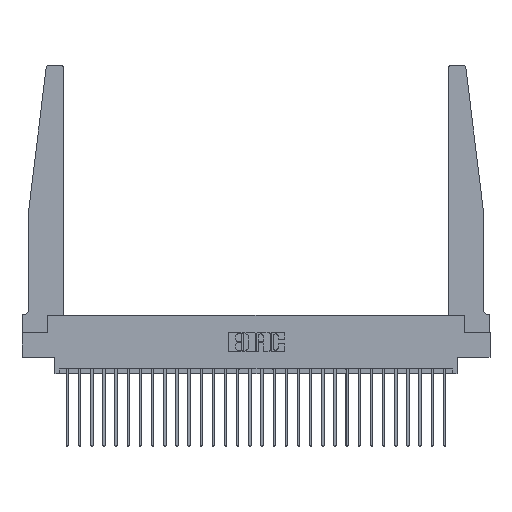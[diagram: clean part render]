
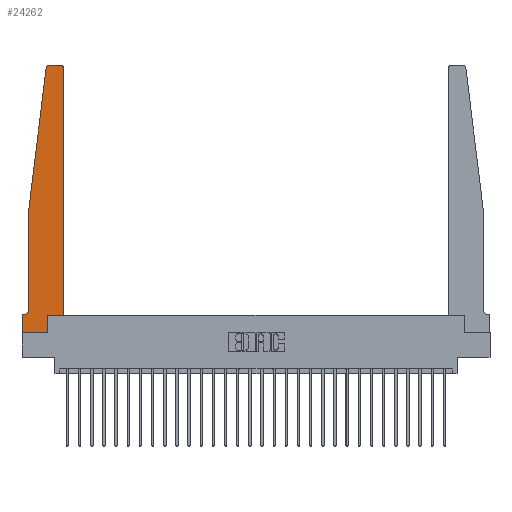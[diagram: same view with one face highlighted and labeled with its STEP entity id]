
A CAD part, top view. The second image highlights one B-rep face of the part: STEP entity #24262.
In plain terms, the highlighted planar face has unit normal (0, 0, 1).
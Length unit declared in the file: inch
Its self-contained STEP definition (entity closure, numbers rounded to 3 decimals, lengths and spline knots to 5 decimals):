
#16 = VECTOR ( 'NONE', #968, 39.37008 ) ;
#245 = ORIENTED_EDGE ( 'NONE', *, *, #18669, .T. ) ;
#570 = CARTESIAN_POINT ( 'NONE',  ( 0., 0.1875, 0.37 ) ) ;
#968 = DIRECTION ( 'NONE',  ( -1., 0., 0. ) ) ;
#1078 = DIRECTION ( 'NONE',  ( 0., 0., 1. ) ) ;
#1541 = EDGE_CURVE ( 'NONE', #19103, #9141, #2400, .T. ) ;
#1894 = AXIS2_PLACEMENT_3D ( 'NONE', #19798, #25999, #13683 ) ;
#2400 = CIRCLE ( 'NONE', #21266, 0.03 ) ;
#2413 = CARTESIAN_POINT ( 'NONE',  ( 0.25, 2.75, 0.37 ) ) ;
#2442 = VERTEX_POINT ( 'NONE', #22703 ) ;
#3156 = DIRECTION ( 'NONE',  ( 1., 0., 0. ) ) ;
#3235 = CARTESIAN_POINT ( 'NONE',  ( 0.24675, 2.72367, 0.37 ) ) ;
#3827 = EDGE_CURVE ( 'NONE', #9141, #15737, #21683, .T. ) ;
#3898 = CARTESIAN_POINT ( 'NONE',  ( 0.2605, 0., 0.37 ) ) ;
#4085 = EDGE_CURVE ( 'NONE', #26745, #8663, #15568, .T. ) ;
#4183 = DIRECTION ( 'NONE',  ( -0.122, -0.992, 0. ) ) ;
#4343 = CARTESIAN_POINT ( 'NONE',  ( 0.2605, 0.18, 0.37 ) ) ;
#4502 = CARTESIAN_POINT ( 'NONE',  ( 0.425, 2.72, 0.37 ) ) ;
#5671 = LINE ( 'NONE', #17486, #16897 ) ;
#5721 = LINE ( 'NONE', #9455, #16 ) ;
#5903 = ORIENTED_EDGE ( 'NONE', *, *, #18547, .T. ) ;
#5923 = DIRECTION ( 'NONE',  ( 0., 1., 0. ) ) ;
#6392 = CIRCLE ( 'NONE', #7645, 0.03 ) ;
#6800 = LINE ( 'NONE', #22717, #17331 ) ;
#6973 = ORIENTED_EDGE ( 'NONE', *, *, #26012, .T. ) ;
#7596 = CARTESIAN_POINT ( 'NONE',  ( 0.015, 0.1875, 0.37 ) ) ;
#7645 = AXIS2_PLACEMENT_3D ( 'NONE', #13870, #1078, #15932 ) ;
#7920 = VERTEX_POINT ( 'NONE', #7596 ) ;
#8250 = VERTEX_POINT ( 'NONE', #570 ) ;
#8261 = ORIENTED_EDGE ( 'NONE', *, *, #21760, .T. ) ;
#8498 = CARTESIAN_POINT ( 'NONE',  ( 0.425, 0.18, 0.37 ) ) ;
#8663 = VERTEX_POINT ( 'NONE', #3898 ) ;
#8764 = ORIENTED_EDGE ( 'NONE', *, *, #1541, .T. ) ;
#9141 = VERTEX_POINT ( 'NONE', #3235 ) ;
#9455 = CARTESIAN_POINT ( 'NONE',  ( 0.065, 0.1875, 0.37 ) ) ;
#10254 = CARTESIAN_POINT ( 'NONE',  ( 0.015, 0.2375, 0.37 ) ) ;
#10686 = CARTESIAN_POINT ( 'NONE',  ( 0.27653, 2.75, 0.37 ) ) ;
#10885 = CARTESIAN_POINT ( 'NONE',  ( 0.27653, 2.72, 0.37 ) ) ;
#11452 = DIRECTION ( 'NONE',  ( 1., 0., 0. ) ) ;
#11508 = CIRCLE ( 'NONE', #18400, 0.05 ) ;
#12431 = DIRECTION ( 'NONE',  ( -1., 0., 0. ) ) ;
#12466 = ORIENTED_EDGE ( 'NONE', *, *, #22343, .T. ) ;
#13050 = DIRECTION ( 'NONE',  ( 1., 0., 0. ) ) ;
#13594 = PLANE ( 'NONE',  #1894 ) ;
#13683 = DIRECTION ( 'NONE',  ( 1., 0., 0. ) ) ;
#13870 = CARTESIAN_POINT ( 'NONE',  ( 0.395, 2.72, 0.37 ) ) ;
#14875 = CARTESIAN_POINT ( 'NONE',  ( 0., 0., 0.37 ) ) ;
#14983 = FACE_OUTER_BOUND ( 'NONE', #15873, .T. ) ;
#15137 = EDGE_CURVE ( 'NONE', #8663, #21943, #17729, .T. ) ;
#15356 = VERTEX_POINT ( 'NONE', #4502 ) ;
#15396 = VERTEX_POINT ( 'NONE', #25438 ) ;
#15483 = VERTEX_POINT ( 'NONE', #17427 ) ;
#15568 = LINE ( 'NONE', #21806, #25865 ) ;
#15737 = VERTEX_POINT ( 'NONE', #18316 ) ;
#15836 = EDGE_CURVE ( 'NONE', #2442, #7920, #11508, .T. ) ;
#15873 = EDGE_LOOP ( 'NONE', ( #12466, #8764, #18384, #8261, #27133, #19035, #5903, #25415, #20415, #245, #6973, #24952 ) ) ;
#15932 = DIRECTION ( 'NONE',  ( 1., 0., 0. ) ) ;
#16013 = LINE ( 'NONE', #2413, #25678 ) ;
#16555 = DIRECTION ( 'NONE',  ( 0., -1., 0. ) ) ;
#16897 = VECTOR ( 'NONE', #21649, 39.37008 ) ;
#17192 = DIRECTION ( 'NONE',  ( -1., 0., 0. ) ) ;
#17331 = VECTOR ( 'NONE', #16555, 39.37008 ) ;
#17427 = CARTESIAN_POINT ( 'NONE',  ( 0.425, 0.18, 0.37 ) ) ;
#17486 = CARTESIAN_POINT ( 'NONE',  ( 0., 0., 0.37 ) ) ;
#17596 = EDGE_CURVE ( 'NONE', #7920, #8250, #5721, .T. ) ;
#17729 = LINE ( 'NONE', #24734, #22582 ) ;
#18316 = CARTESIAN_POINT ( 'NONE',  ( 0.065, 1.25, 0.37 ) ) ;
#18384 = ORIENTED_EDGE ( 'NONE', *, *, #3827, .T. ) ;
#18400 = AXIS2_PLACEMENT_3D ( 'NONE', #10254, #24796, #12431 ) ;
#18516 = VECTOR ( 'NONE', #3156, 39.37008 ) ;
#18547 = EDGE_CURVE ( 'NONE', #8250, #26745, #5671, .T. ) ;
#18669 = EDGE_CURVE ( 'NONE', #21943, #15483, #24626, .T. ) ;
#19035 = ORIENTED_EDGE ( 'NONE', *, *, #17596, .T. ) ;
#19103 = VERTEX_POINT ( 'NONE', #10686 ) ;
#19274 = VECTOR ( 'NONE', #23130, 39.37008 ) ;
#19798 = CARTESIAN_POINT ( 'NONE',  ( 0., 0.1875, 0.37 ) ) ;
#20415 = ORIENTED_EDGE ( 'NONE', *, *, #15137, .T. ) ;
#21038 = VECTOR ( 'NONE', #4183, 39.37008 ) ;
#21266 = AXIS2_PLACEMENT_3D ( 'NONE', #10885, #25394, #13050 ) ;
#21649 = DIRECTION ( 'NONE',  ( 0., -1., 0. ) ) ;
#21683 = LINE ( 'NONE', #25129, #21038 ) ;
#21760 = EDGE_CURVE ( 'NONE', #15737, #2442, #6800, .T. ) ;
#21806 = CARTESIAN_POINT ( 'NONE',  ( 0., 0., 0.37 ) ) ;
#21943 = VERTEX_POINT ( 'NONE', #4343 ) ;
#22007 = CARTESIAN_POINT ( 'NONE',  ( 0.425, 0.18, 0.37 ) ) ;
#22343 = EDGE_CURVE ( 'NONE', #15396, #19103, #16013, .T. ) ;
#22582 = VECTOR ( 'NONE', #5923, 39.37008 ) ;
#22703 = CARTESIAN_POINT ( 'NONE',  ( 0.065, 0.2375, 0.37 ) ) ;
#22717 = CARTESIAN_POINT ( 'NONE',  ( 0.065, 1.25, 0.37 ) ) ;
#23130 = DIRECTION ( 'NONE',  ( 0., 1., 0. ) ) ;
#24262 = ADVANCED_FACE ( 'NONE', ( #14983 ), #13594, .T. ) ;
#24626 = LINE ( 'NONE', #22007, #18516 ) ;
#24734 = CARTESIAN_POINT ( 'NONE',  ( 0.2605, 0.18, 0.37 ) ) ;
#24744 = LINE ( 'NONE', #8498, #19274 ) ;
#24796 = DIRECTION ( 'NONE',  ( 0., 0., -1. ) ) ;
#24952 = ORIENTED_EDGE ( 'NONE', *, *, #27045, .T. ) ;
#25129 = CARTESIAN_POINT ( 'NONE',  ( 0.065, 1.25, 0.37 ) ) ;
#25394 = DIRECTION ( 'NONE',  ( 0., 0., 1. ) ) ;
#25415 = ORIENTED_EDGE ( 'NONE', *, *, #4085, .T. ) ;
#25438 = CARTESIAN_POINT ( 'NONE',  ( 0.395, 2.75, 0.37 ) ) ;
#25678 = VECTOR ( 'NONE', #17192, 39.37008 ) ;
#25865 = VECTOR ( 'NONE', #11452, 39.37008 ) ;
#25999 = DIRECTION ( 'NONE',  ( 0., 0., 1. ) ) ;
#26012 = EDGE_CURVE ( 'NONE', #15483, #15356, #24744, .T. ) ;
#26745 = VERTEX_POINT ( 'NONE', #14875 ) ;
#27045 = EDGE_CURVE ( 'NONE', #15356, #15396, #6392, .T. ) ;
#27133 = ORIENTED_EDGE ( 'NONE', *, *, #15836, .T. ) ;
